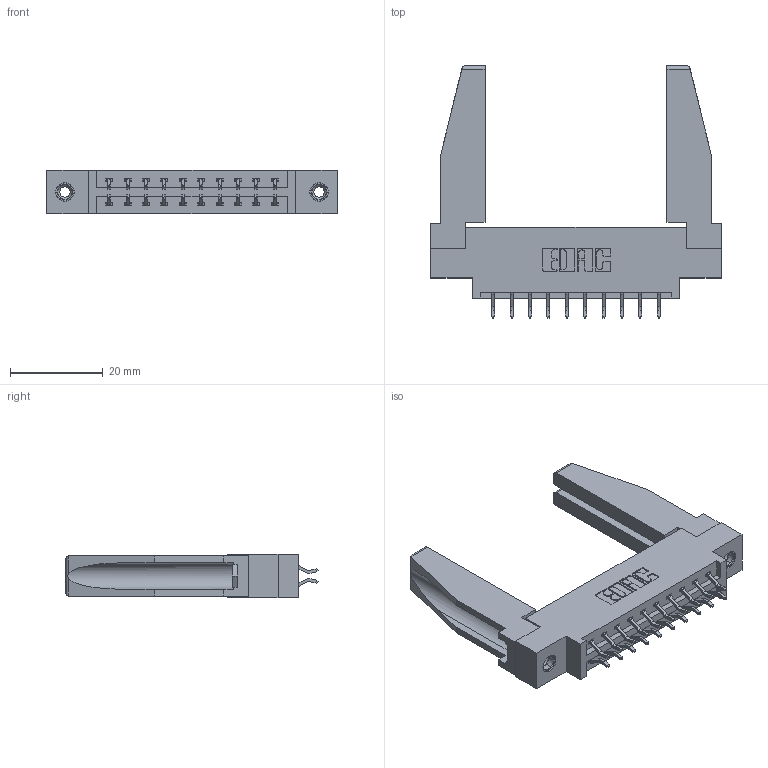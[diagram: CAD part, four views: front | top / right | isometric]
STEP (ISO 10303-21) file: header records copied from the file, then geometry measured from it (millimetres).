
FILE_DESCRIPTION (( 'STEP AP203' ), '1' );
FILE_NAME ('337-020-556-878.STEP', '2019-10-10T19:39:02', ( '' ), ( '' ), 'SwSTEP 2.0', 'SolidWorks 2016', '' );
FILE_SCHEMA (( 'CONFIG_CONTROL_DESIGN' ));
Length unit declared in the file: inch
Products named in the file (5): 307-220-078; 345-250-001_345-250-001-102; 337-020-556-878; 337 Part_0.170 Offset - 0.156 Dia-TI; 345-292-001_556 Tail
Assembly tree (25 placements, depth 2):
  337-020-556-878
    337 Part_0.170 Offset - 0.156 Dia-TI
    345-292-001_556 Tail  x20
    345-250-001_345-250-001-102  x2
    307-220-078  x2
Bounding box: 62.64 x 54.37 x 9.4 mm (x, y, z)
Volume: 10050.2 mm3; surface area: 10453.7 mm2
Topology: 25 solids, 25 shells, 1448 faces, 4233 edges, 2786 vertices
Faces by surface type: plane 998, cylinder 434, cone 12, torus 4
Entity records: 14684 total; most frequent: CARTESIAN_POINT 2516, ORIENTED_EDGE 2396, DIRECTION 2194, EDGE_CURVE 1198, VECTOR 1024, LINE 1024, VERTEX_POINT 792, AXIS2_PLACEMENT_3D 585
